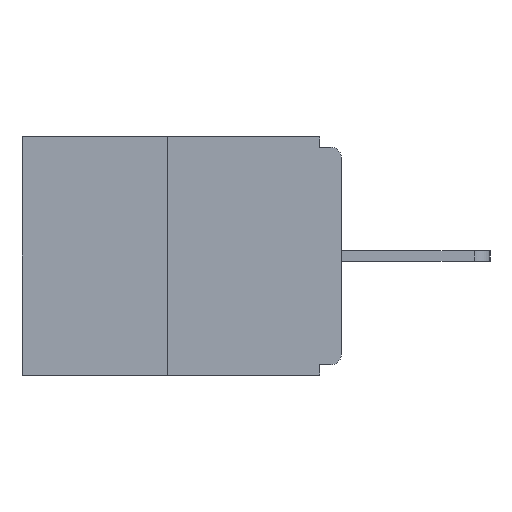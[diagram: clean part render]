
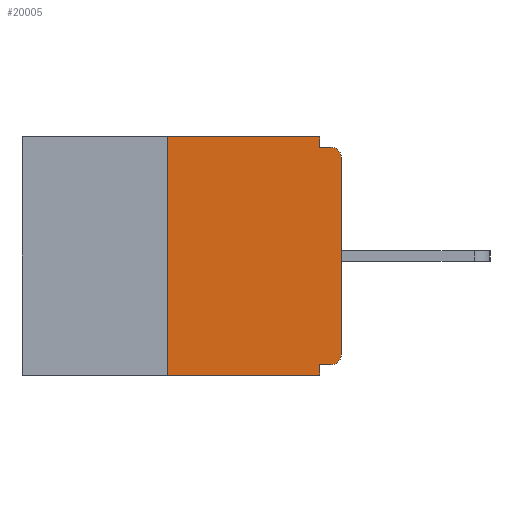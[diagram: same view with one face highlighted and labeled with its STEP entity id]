
A CAD part, left-side view. The second image highlights one B-rep face of the part: STEP entity #20005.
In plain terms, the highlighted planar face has unit normal (-1, 0, 0).
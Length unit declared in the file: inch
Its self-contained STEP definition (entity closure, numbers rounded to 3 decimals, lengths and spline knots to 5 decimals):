
#188 = LINE ( 'NONE', #6232, #7743 ) ;
#199 = DIRECTION ( 'NONE',  ( 0., -1., 0. ) ) ;
#353 = DIRECTION ( 'NONE',  ( 0., 0., -1. ) ) ;
#439 = VERTEX_POINT ( 'NONE', #8014 ) ;
#532 = VERTEX_POINT ( 'NONE', #14838 ) ;
#844 = VERTEX_POINT ( 'NONE', #21773 ) ;
#1941 = ORIENTED_EDGE ( 'NONE', *, *, #14183, .F. ) ;
#1989 = DIRECTION ( 'NONE',  ( -1., 0., 0. ) ) ;
#2284 = CARTESIAN_POINT ( 'NONE',  ( 0., 0.015, -0.313 ) ) ;
#2904 = ORIENTED_EDGE ( 'NONE', *, *, #16162, .F. ) ;
#2943 = DIRECTION ( 'NONE',  ( 0., 0., -1. ) ) ;
#3006 = CARTESIAN_POINT ( 'NONE',  ( 0., 0.015, -0.015 ) ) ;
#3452 = CARTESIAN_POINT ( 'NONE',  ( 0., 0.25, -0.343 ) ) ;
#3468 = EDGE_LOOP ( 'NONE', ( #19456, #13324, #12474, #1941, #16895, #3707, #20346, #11665, #5853, #2904 ) ) ;
#3707 = ORIENTED_EDGE ( 'NONE', *, *, #18709, .T. ) ;
#3758 = DIRECTION ( 'NONE',  ( 0., 0., -1. ) ) ;
#4388 = EDGE_CURVE ( 'NONE', #16899, #10468, #188, .T. ) ;
#4620 = CIRCLE ( 'NONE', #14485, 0.015 ) ;
#5853 = ORIENTED_EDGE ( 'NONE', *, *, #21603, .F. ) ;
#5931 = CARTESIAN_POINT ( 'NONE',  ( 0., 0.46, -0.343 ) ) ;
#6150 = CARTESIAN_POINT ( 'NONE',  ( 0., 0.46, 0. ) ) ;
#6232 = CARTESIAN_POINT ( 'NONE',  ( 0., 0., 0. ) ) ;
#6245 = CARTESIAN_POINT ( 'NONE',  ( 0., 0.46, 0. ) ) ;
#6393 = DIRECTION ( 'NONE',  ( 1., 0., 0. ) ) ;
#6908 = CARTESIAN_POINT ( 'NONE',  ( 0., 0.031, 0. ) ) ;
#7257 = CARTESIAN_POINT ( 'NONE',  ( 0., 0.015, -0.328 ) ) ;
#7358 = EDGE_CURVE ( 'NONE', #17672, #844, #10067, .T. ) ;
#7691 = VECTOR ( 'NONE', #199, 39.37008 ) ;
#7743 = VECTOR ( 'NONE', #10086, 39.37008 ) ;
#7931 = DIRECTION ( 'NONE',  ( 0., -1., 0. ) ) ;
#7955 = DIRECTION ( 'NONE',  ( 0., 0., -1. ) ) ;
#7992 = DIRECTION ( 'NONE',  ( 0., -1., 0. ) ) ;
#8012 = CARTESIAN_POINT ( 'NONE',  ( 0., 0.25, 0. ) ) ;
#8014 = CARTESIAN_POINT ( 'NONE',  ( 0., 0.031, 0. ) ) ;
#8346 = CARTESIAN_POINT ( 'NONE',  ( 0., 0., -0.328 ) ) ;
#8725 = LINE ( 'NONE', #6908, #14061 ) ;
#10067 = LINE ( 'NONE', #8012, #22888 ) ;
#10086 = DIRECTION ( 'NONE',  ( 0., 0., 1. ) ) ;
#10421 = VECTOR ( 'NONE', #19922, 39.37008 ) ;
#10468 = VERTEX_POINT ( 'NONE', #15914 ) ;
#10561 = AXIS2_PLACEMENT_3D ( 'NONE', #2284, #15912, #7955 ) ;
#10984 = CIRCLE ( 'NONE', #10561, 0.015 ) ;
#11665 = ORIENTED_EDGE ( 'NONE', *, *, #15097, .T. ) ;
#12058 = LINE ( 'NONE', #17935, #25450 ) ;
#12474 = ORIENTED_EDGE ( 'NONE', *, *, #13028, .T. ) ;
#12571 = CARTESIAN_POINT ( 'NONE',  ( 0., 0.031, -0.328 ) ) ;
#13028 = EDGE_CURVE ( 'NONE', #17672, #532, #23461, .T. ) ;
#13324 = ORIENTED_EDGE ( 'NONE', *, *, #7358, .F. ) ;
#13405 = LINE ( 'NONE', #21262, #15277 ) ;
#14061 = VECTOR ( 'NONE', #2943, 39.37008 ) ;
#14183 = EDGE_CURVE ( 'NONE', #24362, #532, #13405, .T. ) ;
#14485 = AXIS2_PLACEMENT_3D ( 'NONE', #17531, #1989, #16939 ) ;
#14838 = CARTESIAN_POINT ( 'NONE',  ( 0., 0.031, -0.343 ) ) ;
#15089 = AXIS2_PLACEMENT_3D ( 'NONE', #6150, #6393, #353 ) ;
#15097 = EDGE_CURVE ( 'NONE', #10468, #22216, #4620, .T. ) ;
#15123 = VERTEX_POINT ( 'NONE', #23369 ) ;
#15277 = VECTOR ( 'NONE', #3758, 39.37008 ) ;
#15912 = DIRECTION ( 'NONE',  ( -1., 0., 0. ) ) ;
#15914 = CARTESIAN_POINT ( 'NONE',  ( 0., 0., -0.03 ) ) ;
#15936 = LINE ( 'NONE', #8346, #10421 ) ;
#16162 = EDGE_CURVE ( 'NONE', #439, #15123, #8725, .T. ) ;
#16282 = PLANE ( 'NONE',  #15089 ) ;
#16895 = ORIENTED_EDGE ( 'NONE', *, *, #17330, .F. ) ;
#16899 = VERTEX_POINT ( 'NONE', #23630 ) ;
#16939 = DIRECTION ( 'NONE',  ( 0., 0., -1. ) ) ;
#17330 = EDGE_CURVE ( 'NONE', #24981, #24362, #15936, .T. ) ;
#17531 = CARTESIAN_POINT ( 'NONE',  ( 0., 0.015, -0.03 ) ) ;
#17672 = VERTEX_POINT ( 'NONE', #3452 ) ;
#17815 = LINE ( 'NONE', #6245, #7691 ) ;
#17903 = DIRECTION ( 'NONE',  ( 0., 0., 1. ) ) ;
#17935 = CARTESIAN_POINT ( 'NONE',  ( 0., 0., -0.015 ) ) ;
#17963 = FACE_OUTER_BOUND ( 'NONE', #3468, .T. ) ;
#18709 = EDGE_CURVE ( 'NONE', #24981, #16899, #10984, .T. ) ;
#19327 = VECTOR ( 'NONE', #7992, 39.37008 ) ;
#19456 = ORIENTED_EDGE ( 'NONE', *, *, #20451, .F. ) ;
#19922 = DIRECTION ( 'NONE',  ( 0., 1., 0. ) ) ;
#20005 = ADVANCED_FACE ( 'NONE', ( #17963 ), #16282, .F. ) ;
#20346 = ORIENTED_EDGE ( 'NONE', *, *, #4388, .T. ) ;
#20451 = EDGE_CURVE ( 'NONE', #844, #439, #17815, .T. ) ;
#21262 = CARTESIAN_POINT ( 'NONE',  ( 0., 0.031, -0.343 ) ) ;
#21603 = EDGE_CURVE ( 'NONE', #15123, #22216, #12058, .T. ) ;
#21773 = CARTESIAN_POINT ( 'NONE',  ( 0., 0.25, 0. ) ) ;
#22216 = VERTEX_POINT ( 'NONE', #3006 ) ;
#22888 = VECTOR ( 'NONE', #17903, 39.37008 ) ;
#23369 = CARTESIAN_POINT ( 'NONE',  ( 0., 0.031, -0.015 ) ) ;
#23461 = LINE ( 'NONE', #5931, #19327 ) ;
#23630 = CARTESIAN_POINT ( 'NONE',  ( 0., 0., -0.313 ) ) ;
#24362 = VERTEX_POINT ( 'NONE', #12571 ) ;
#24981 = VERTEX_POINT ( 'NONE', #7257 ) ;
#25450 = VECTOR ( 'NONE', #7931, 39.37008 ) ;
